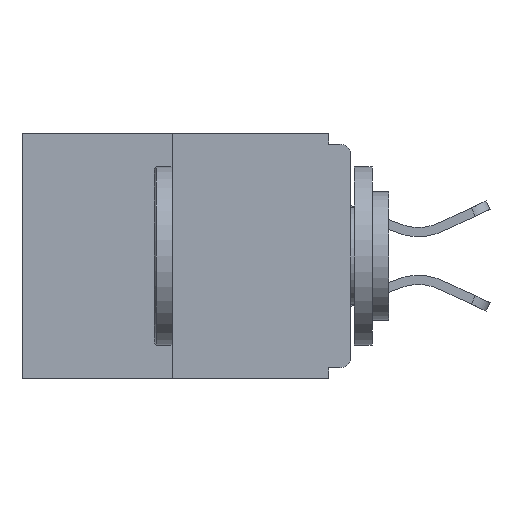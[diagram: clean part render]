
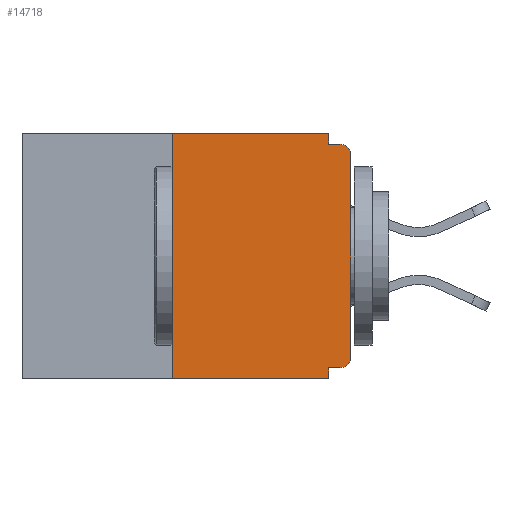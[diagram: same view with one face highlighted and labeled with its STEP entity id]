
A CAD part, left-side view. The second image highlights one B-rep face of the part: STEP entity #14718.
In plain terms, the highlighted planar face has unit normal (-1, 0, 0).
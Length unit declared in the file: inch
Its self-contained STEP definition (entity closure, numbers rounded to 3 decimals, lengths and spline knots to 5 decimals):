
#33 = VERTEX_POINT ( 'NONE', #6345 ) ;
#439 = DIRECTION ( 'NONE',  ( -1., 0., 0. ) ) ;
#740 = DIRECTION ( 'NONE',  ( 0., 1., 0. ) ) ;
#751 = CARTESIAN_POINT ( 'NONE',  ( 0., 0.015, -0.03 ) ) ;
#1213 = CARTESIAN_POINT ( 'NONE',  ( 0., 0.015, -0.313 ) ) ;
#1973 = AXIS2_PLACEMENT_3D ( 'NONE', #751, #439, #13096 ) ;
#2819 = CARTESIAN_POINT ( 'NONE',  ( 0., 0., -0.328 ) ) ;
#3101 = LINE ( 'NONE', #17878, #11370 ) ;
#3825 = DIRECTION ( 'NONE',  ( 0., 0., -1. ) ) ;
#3959 = CARTESIAN_POINT ( 'NONE',  ( 0., 0.015, -0.328 ) ) ;
#3985 = DIRECTION ( 'NONE',  ( 0., 0., -1. ) ) ;
#4212 = EDGE_CURVE ( 'NONE', #26702, #33, #12148, .T. ) ;
#4317 = EDGE_CURVE ( 'NONE', #24605, #15502, #3101, .T. ) ;
#4329 = CARTESIAN_POINT ( 'NONE',  ( 0., 0.031, 0. ) ) ;
#4407 = PLANE ( 'NONE',  #19392 ) ;
#5048 = VECTOR ( 'NONE', #740, 39.37008 ) ;
#5304 = VECTOR ( 'NONE', #18754, 39.37008 ) ;
#6345 = CARTESIAN_POINT ( 'NONE',  ( 0., 0.031, 0. ) ) ;
#6505 = ORIENTED_EDGE ( 'NONE', *, *, #10792, .T. ) ;
#6555 = DIRECTION ( 'NONE',  ( 0., -1., 0. ) ) ;
#6614 = CARTESIAN_POINT ( 'NONE',  ( 0., 0., -0.03 ) ) ;
#7318 = LINE ( 'NONE', #11291, #5304 ) ;
#7632 = ORIENTED_EDGE ( 'NONE', *, *, #17258, .F. ) ;
#7803 = LINE ( 'NONE', #24093, #15174 ) ;
#9346 = CARTESIAN_POINT ( 'NONE',  ( 0., 0.46, 0. ) ) ;
#9387 = LINE ( 'NONE', #2819, #5048 ) ;
#9403 = ORIENTED_EDGE ( 'NONE', *, *, #4212, .F. ) ;
#10055 = EDGE_CURVE ( 'NONE', #15502, #25629, #22658, .T. ) ;
#10241 = EDGE_CURVE ( 'NONE', #13505, #25629, #25386, .T. ) ;
#10400 = VERTEX_POINT ( 'NONE', #13075 ) ;
#10587 = VECTOR ( 'NONE', #15343, 39.37008 ) ;
#10792 = EDGE_CURVE ( 'NONE', #14495, #10400, #7318, .T. ) ;
#11291 = CARTESIAN_POINT ( 'NONE',  ( 0., 0.46, -0.343 ) ) ;
#11370 = VECTOR ( 'NONE', #15146, 39.37008 ) ;
#11398 = AXIS2_PLACEMENT_3D ( 'NONE', #1213, #23804, #3825 ) ;
#11435 = ORIENTED_EDGE ( 'NONE', *, *, #17111, .F. ) ;
#12073 = DIRECTION ( 'NONE',  ( 0., 0., -1. ) ) ;
#12148 = LINE ( 'NONE', #13080, #10587 ) ;
#13017 = LINE ( 'NONE', #31149, #26708 ) ;
#13075 = CARTESIAN_POINT ( 'NONE',  ( 0., 0.031, -0.343 ) ) ;
#13080 = CARTESIAN_POINT ( 'NONE',  ( 0., 0.46, 0. ) ) ;
#13096 = DIRECTION ( 'NONE',  ( 0., 0., -1. ) ) ;
#13493 = DIRECTION ( 'NONE',  ( 0., 0., 1. ) ) ;
#13505 = VERTEX_POINT ( 'NONE', #19313 ) ;
#13999 = CARTESIAN_POINT ( 'NONE',  ( 0., 0., -0.313 ) ) ;
#14114 = EDGE_LOOP ( 'NONE', ( #9403, #23285, #6505, #11435, #24002, #29532, #18815, #20265, #24721, #7632 ) ) ;
#14448 = VECTOR ( 'NONE', #6555, 39.37008 ) ;
#14495 = VERTEX_POINT ( 'NONE', #30796 ) ;
#14718 = ADVANCED_FACE ( 'NONE', ( #20261 ), #4407, .F. ) ;
#14761 = CARTESIAN_POINT ( 'NONE',  ( 0., 0.031, -0.328 ) ) ;
#15146 = DIRECTION ( 'NONE',  ( 0., 0., 1. ) ) ;
#15174 = VECTOR ( 'NONE', #3985, 39.37008 ) ;
#15343 = DIRECTION ( 'NONE',  ( 0., -1., 0. ) ) ;
#15502 = VERTEX_POINT ( 'NONE', #6614 ) ;
#16631 = VERTEX_POINT ( 'NONE', #14761 ) ;
#17111 = EDGE_CURVE ( 'NONE', #16631, #10400, #7803, .T. ) ;
#17258 = EDGE_CURVE ( 'NONE', #33, #13505, #29642, .T. ) ;
#17878 = CARTESIAN_POINT ( 'NONE',  ( 0., 0., 0. ) ) ;
#18754 = DIRECTION ( 'NONE',  ( 0., -1., 0. ) ) ;
#18815 = ORIENTED_EDGE ( 'NONE', *, *, #4317, .T. ) ;
#19313 = CARTESIAN_POINT ( 'NONE',  ( 0., 0.031, -0.015 ) ) ;
#19392 = AXIS2_PLACEMENT_3D ( 'NONE', #9346, #27009, #12073 ) ;
#20261 = FACE_OUTER_BOUND ( 'NONE', #14114, .T. ) ;
#20265 = ORIENTED_EDGE ( 'NONE', *, *, #10055, .T. ) ;
#21611 = EDGE_CURVE ( 'NONE', #32136, #24605, #27428, .T. ) ;
#22545 = VECTOR ( 'NONE', #24430, 39.37008 ) ;
#22658 = CIRCLE ( 'NONE', #1973, 0.015 ) ;
#23285 = ORIENTED_EDGE ( 'NONE', *, *, #28857, .F. ) ;
#23804 = DIRECTION ( 'NONE',  ( -1., 0., 0. ) ) ;
#24002 = ORIENTED_EDGE ( 'NONE', *, *, #25569, .F. ) ;
#24093 = CARTESIAN_POINT ( 'NONE',  ( 0., 0.031, -0.343 ) ) ;
#24430 = DIRECTION ( 'NONE',  ( 0., 0., -1. ) ) ;
#24605 = VERTEX_POINT ( 'NONE', #13999 ) ;
#24721 = ORIENTED_EDGE ( 'NONE', *, *, #10241, .F. ) ;
#25386 = LINE ( 'NONE', #26307, #14448 ) ;
#25518 = CARTESIAN_POINT ( 'NONE',  ( 0., 0.015, -0.015 ) ) ;
#25569 = EDGE_CURVE ( 'NONE', #32136, #16631, #9387, .T. ) ;
#25629 = VERTEX_POINT ( 'NONE', #25518 ) ;
#26307 = CARTESIAN_POINT ( 'NONE',  ( 0., 0., -0.015 ) ) ;
#26702 = VERTEX_POINT ( 'NONE', #28965 ) ;
#26708 = VECTOR ( 'NONE', #13493, 39.37008 ) ;
#27009 = DIRECTION ( 'NONE',  ( 1., 0., 0. ) ) ;
#27428 = CIRCLE ( 'NONE', #11398, 0.015 ) ;
#28857 = EDGE_CURVE ( 'NONE', #14495, #26702, #13017, .T. ) ;
#28965 = CARTESIAN_POINT ( 'NONE',  ( 0., 0.25, 0. ) ) ;
#29532 = ORIENTED_EDGE ( 'NONE', *, *, #21611, .T. ) ;
#29642 = LINE ( 'NONE', #4329, #22545 ) ;
#30796 = CARTESIAN_POINT ( 'NONE',  ( 0., 0.25, -0.343 ) ) ;
#31149 = CARTESIAN_POINT ( 'NONE',  ( 0., 0.25, 0. ) ) ;
#32136 = VERTEX_POINT ( 'NONE', #3959 ) ;
